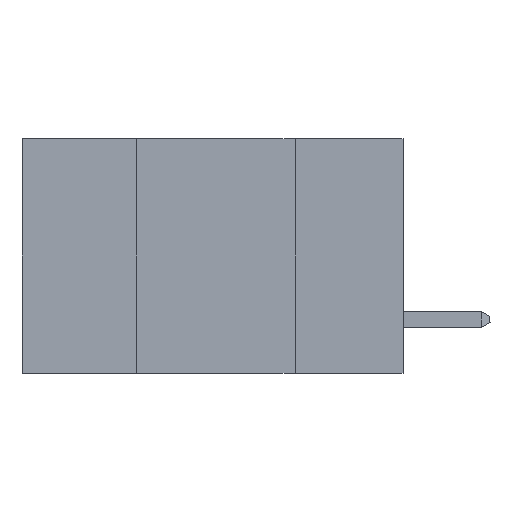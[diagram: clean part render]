
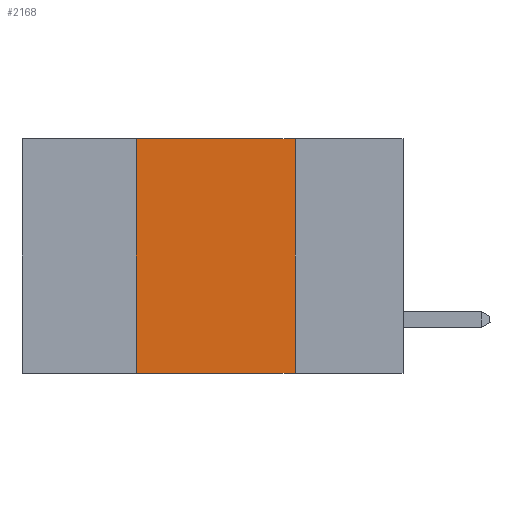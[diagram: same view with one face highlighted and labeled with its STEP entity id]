
A CAD part, left-side view. The second image highlights one B-rep face of the part: STEP entity #2168.
In plain terms, the highlighted planar face has unit normal (-1, 0, 0).
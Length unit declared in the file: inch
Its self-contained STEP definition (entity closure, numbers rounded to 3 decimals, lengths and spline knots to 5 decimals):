
#508 = CARTESIAN_POINT ( 'NONE',  ( 0., 0.6, -0.37 ) ) ;
#1097 = VECTOR ( 'NONE', #11702, 39.37008 ) ;
#1574 = EDGE_CURVE ( 'NONE', #12710, #5066, #13811, .T. ) ;
#1787 = VECTOR ( 'NONE', #10282, 39.37008 ) ;
#2004 = CARTESIAN_POINT ( 'NONE',  ( 0., 0.17, 0. ) ) ;
#2168 = ADVANCED_FACE ( 'NONE', ( #6806 ), #8949, .F. ) ;
#2214 = EDGE_CURVE ( 'NONE', #12710, #4637, #5405, .T. ) ;
#2310 = CARTESIAN_POINT ( 'NONE',  ( 0., 0.6, 0. ) ) ;
#3110 = EDGE_LOOP ( 'NONE', ( #3634, #11575, #10494, #10154 ) ) ;
#3248 = DIRECTION ( 'NONE',  ( 1., 0., 0. ) ) ;
#3261 = CARTESIAN_POINT ( 'NONE',  ( 0., 0.17, -0.37 ) ) ;
#3302 = DIRECTION ( 'NONE',  ( 0., -1., 0. ) ) ;
#3634 = ORIENTED_EDGE ( 'NONE', *, *, #4550, .F. ) ;
#4550 = EDGE_CURVE ( 'NONE', #7067, #5066, #8942, .T. ) ;
#4637 = VERTEX_POINT ( 'NONE', #5759 ) ;
#4753 = AXIS2_PLACEMENT_3D ( 'NONE', #2310, #3248, #11061 ) ;
#4857 = LINE ( 'NONE', #7842, #12523 ) ;
#5066 = VERTEX_POINT ( 'NONE', #3261 ) ;
#5405 = LINE ( 'NONE', #12357, #1787 ) ;
#5759 = CARTESIAN_POINT ( 'NONE',  ( 0., 0.42, 0. ) ) ;
#6806 = FACE_OUTER_BOUND ( 'NONE', #3110, .T. ) ;
#7037 = EDGE_CURVE ( 'NONE', #4637, #7067, #4857, .T. ) ;
#7067 = VERTEX_POINT ( 'NONE', #13289 ) ;
#7717 = DIRECTION ( 'NONE',  ( 0., 0., -1. ) ) ;
#7842 = CARTESIAN_POINT ( 'NONE',  ( 0., 0.6, 0. ) ) ;
#8942 = LINE ( 'NONE', #2004, #12775 ) ;
#8949 = PLANE ( 'NONE',  #4753 ) ;
#10118 = CARTESIAN_POINT ( 'NONE',  ( 0., 0.42, -0.37 ) ) ;
#10154 = ORIENTED_EDGE ( 'NONE', *, *, #1574, .T. ) ;
#10282 = DIRECTION ( 'NONE',  ( 0., 0., 1. ) ) ;
#10494 = ORIENTED_EDGE ( 'NONE', *, *, #2214, .F. ) ;
#11061 = DIRECTION ( 'NONE',  ( 0., 0., -1. ) ) ;
#11575 = ORIENTED_EDGE ( 'NONE', *, *, #7037, .F. ) ;
#11702 = DIRECTION ( 'NONE',  ( 0., -1., 0. ) ) ;
#12357 = CARTESIAN_POINT ( 'NONE',  ( 0., 0.42, 0. ) ) ;
#12523 = VECTOR ( 'NONE', #3302, 39.37008 ) ;
#12710 = VERTEX_POINT ( 'NONE', #10118 ) ;
#12775 = VECTOR ( 'NONE', #7717, 39.37008 ) ;
#13289 = CARTESIAN_POINT ( 'NONE',  ( 0., 0.17, 0. ) ) ;
#13811 = LINE ( 'NONE', #508, #1097 ) ;
